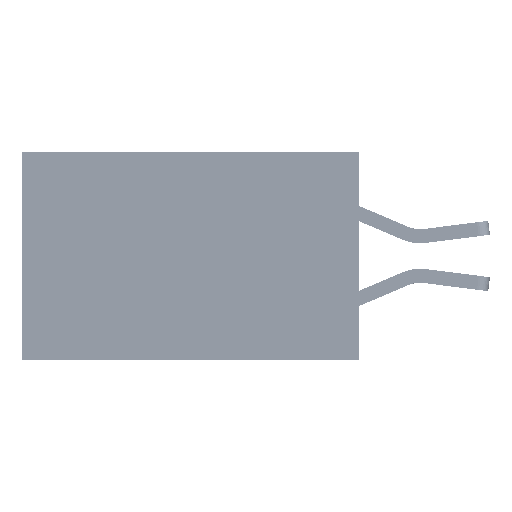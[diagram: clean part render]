
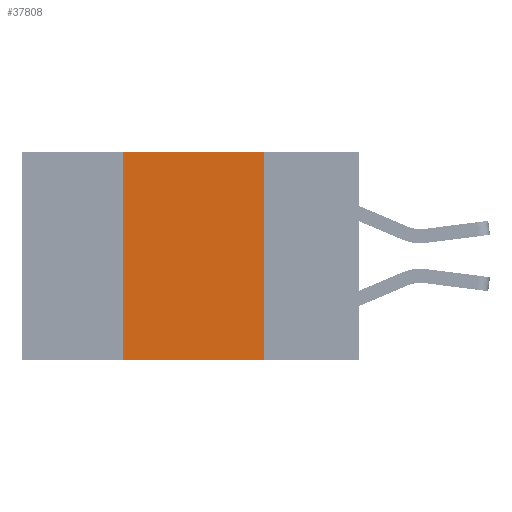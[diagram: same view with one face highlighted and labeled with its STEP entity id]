
A CAD part, left-side view. The second image highlights one B-rep face of the part: STEP entity #37808.
In plain terms, the highlighted planar face has unit normal (-1, 0, 0).
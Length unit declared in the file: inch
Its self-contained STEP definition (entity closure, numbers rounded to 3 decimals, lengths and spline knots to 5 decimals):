
#1557 = VECTOR ( 'NONE', #46121, 39.37008 ) ;
#5934 = DIRECTION ( 'NONE',  ( 0., 0., 1. ) ) ;
#6138 = EDGE_CURVE ( 'NONE', #38385, #23945, #26091, .T. ) ;
#6315 = VECTOR ( 'NONE', #5934, 39.37008 ) ;
#6443 = EDGE_CURVE ( 'NONE', #18762, #23945, #16919, .T. ) ;
#11447 = EDGE_CURVE ( 'NONE', #28887, #38385, #34055, .T. ) ;
#12477 = CARTESIAN_POINT ( 'NONE',  ( 0., 0.42, 0. ) ) ;
#13272 = ORIENTED_EDGE ( 'NONE', *, *, #34502, .F. ) ;
#14916 = ORIENTED_EDGE ( 'NONE', *, *, #6443, .T. ) ;
#16919 = LINE ( 'NONE', #44265, #33866 ) ;
#18021 = CARTESIAN_POINT ( 'NONE',  ( 0., 0.17, 0. ) ) ;
#18417 = DIRECTION ( 'NONE',  ( 0., 0., -1. ) ) ;
#18762 = VERTEX_POINT ( 'NONE', #41224 ) ;
#19728 = EDGE_LOOP ( 'NONE', ( #42264, #35922, #13272, #14916 ) ) ;
#22330 = CARTESIAN_POINT ( 'NONE',  ( 0., 0.6, 0. ) ) ;
#23945 = VERTEX_POINT ( 'NONE', #36704 ) ;
#25712 = LINE ( 'NONE', #41593, #6315 ) ;
#26091 = LINE ( 'NONE', #18021, #1557 ) ;
#28138 = DIRECTION ( 'NONE',  ( 0., -1., 0. ) ) ;
#28887 = VERTEX_POINT ( 'NONE', #12477 ) ;
#30669 = CARTESIAN_POINT ( 'NONE',  ( 0., 0.6, 0. ) ) ;
#32477 = CARTESIAN_POINT ( 'NONE',  ( 0., 0.17, 0. ) ) ;
#33866 = VECTOR ( 'NONE', #28138, 39.37008 ) ;
#34055 = LINE ( 'NONE', #30669, #47549 ) ;
#34502 = EDGE_CURVE ( 'NONE', #18762, #28887, #25712, .T. ) ;
#34527 = DIRECTION ( 'NONE',  ( 1., 0., 0. ) ) ;
#35922 = ORIENTED_EDGE ( 'NONE', *, *, #11447, .F. ) ;
#36704 = CARTESIAN_POINT ( 'NONE',  ( 0., 0.17, -0.37 ) ) ;
#37808 = ADVANCED_FACE ( 'NONE', ( #42886 ), #43137, .F. ) ;
#38385 = VERTEX_POINT ( 'NONE', #32477 ) ;
#41224 = CARTESIAN_POINT ( 'NONE',  ( 0., 0.42, -0.37 ) ) ;
#41593 = CARTESIAN_POINT ( 'NONE',  ( 0., 0.42, 0. ) ) ;
#42133 = DIRECTION ( 'NONE',  ( 0., -1., 0. ) ) ;
#42264 = ORIENTED_EDGE ( 'NONE', *, *, #6138, .F. ) ;
#42886 = FACE_OUTER_BOUND ( 'NONE', #19728, .T. ) ;
#43137 = PLANE ( 'NONE',  #47254 ) ;
#44265 = CARTESIAN_POINT ( 'NONE',  ( 0., 0.6, -0.37 ) ) ;
#46121 = DIRECTION ( 'NONE',  ( 0., 0., -1. ) ) ;
#47254 = AXIS2_PLACEMENT_3D ( 'NONE', #22330, #34527, #18417 ) ;
#47549 = VECTOR ( 'NONE', #42133, 39.37008 ) ;
